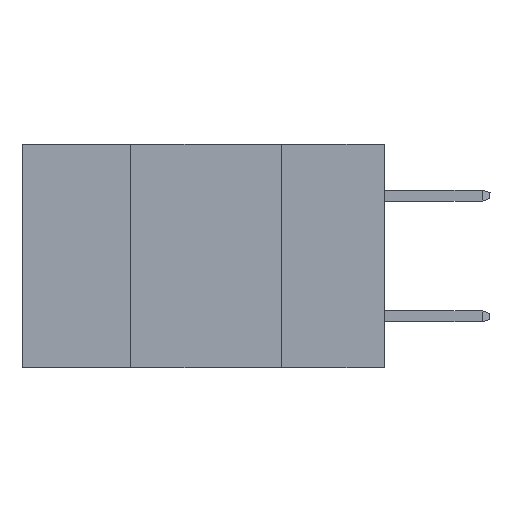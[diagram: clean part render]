
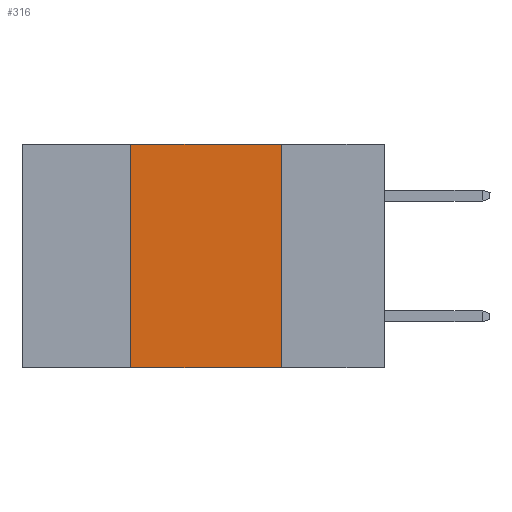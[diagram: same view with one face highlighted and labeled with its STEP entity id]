
A CAD part, left-side view. The second image highlights one B-rep face of the part: STEP entity #316.
In plain terms, the highlighted planar face has unit normal (-1, 0, 0).
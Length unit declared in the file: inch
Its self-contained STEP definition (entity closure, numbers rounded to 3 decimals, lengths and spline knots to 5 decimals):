
#257 = CARTESIAN_POINT ( 'NONE',  ( 0., 0.17, -0.37 ) ) ;
#316 = ADVANCED_FACE ( 'NONE', ( #5950 ), #2032, .F. ) ;
#1661 = DIRECTION ( 'NONE',  ( 0., 0., 1. ) ) ;
#2032 = PLANE ( 'NONE',  #10308 ) ;
#2471 = LINE ( 'NONE', #22151, #26178 ) ;
#4388 = DIRECTION ( 'NONE',  ( 0., 0., -1. ) ) ;
#5950 = FACE_OUTER_BOUND ( 'NONE', #16583, .T. ) ;
#6291 = ORIENTED_EDGE ( 'NONE', *, *, #9419, .F. ) ;
#8715 = CARTESIAN_POINT ( 'NONE',  ( 0., 0.42, 0. ) ) ;
#9419 = EDGE_CURVE ( 'NONE', #11659, #22897, #2471, .T. ) ;
#10308 = AXIS2_PLACEMENT_3D ( 'NONE', #18331, #15590, #4388 ) ;
#10781 = VECTOR ( 'NONE', #28492, 39.37008 ) ;
#11659 = VERTEX_POINT ( 'NONE', #18787 ) ;
#12072 = EDGE_CURVE ( 'NONE', #27499, #22897, #26766, .T. ) ;
#15590 = DIRECTION ( 'NONE',  ( 1., 0., 0. ) ) ;
#15712 = EDGE_CURVE ( 'NONE', #27499, #27342, #17004, .T. ) ;
#16083 = CARTESIAN_POINT ( 'NONE',  ( 0., 0.6, -0.37 ) ) ;
#16583 = EDGE_LOOP ( 'NONE', ( #6291, #23766, #29280, #17885 ) ) ;
#17004 = LINE ( 'NONE', #17456, #25791 ) ;
#17425 = DIRECTION ( 'NONE',  ( 0., 0., -1. ) ) ;
#17456 = CARTESIAN_POINT ( 'NONE',  ( 0., 0.42, 0. ) ) ;
#17885 = ORIENTED_EDGE ( 'NONE', *, *, #12072, .T. ) ;
#18331 = CARTESIAN_POINT ( 'NONE',  ( 0., 0.6, 0. ) ) ;
#18787 = CARTESIAN_POINT ( 'NONE',  ( 0., 0.17, 0. ) ) ;
#19062 = EDGE_CURVE ( 'NONE', #27342, #11659, #25749, .T. ) ;
#22151 = CARTESIAN_POINT ( 'NONE',  ( 0., 0.17, 0. ) ) ;
#22897 = VERTEX_POINT ( 'NONE', #257 ) ;
#23766 = ORIENTED_EDGE ( 'NONE', *, *, #19062, .F. ) ;
#23912 = CARTESIAN_POINT ( 'NONE',  ( 0., 0.6, 0. ) ) ;
#25749 = LINE ( 'NONE', #23912, #10781 ) ;
#25791 = VECTOR ( 'NONE', #1661, 39.37008 ) ;
#26178 = VECTOR ( 'NONE', #17425, 39.37008 ) ;
#26253 = CARTESIAN_POINT ( 'NONE',  ( 0., 0.42, -0.37 ) ) ;
#26398 = VECTOR ( 'NONE', #27297, 39.37008 ) ;
#26766 = LINE ( 'NONE', #16083, #26398 ) ;
#27297 = DIRECTION ( 'NONE',  ( 0., -1., 0. ) ) ;
#27342 = VERTEX_POINT ( 'NONE', #8715 ) ;
#27499 = VERTEX_POINT ( 'NONE', #26253 ) ;
#28492 = DIRECTION ( 'NONE',  ( 0., -1., 0. ) ) ;
#29280 = ORIENTED_EDGE ( 'NONE', *, *, #15712, .F. ) ;
